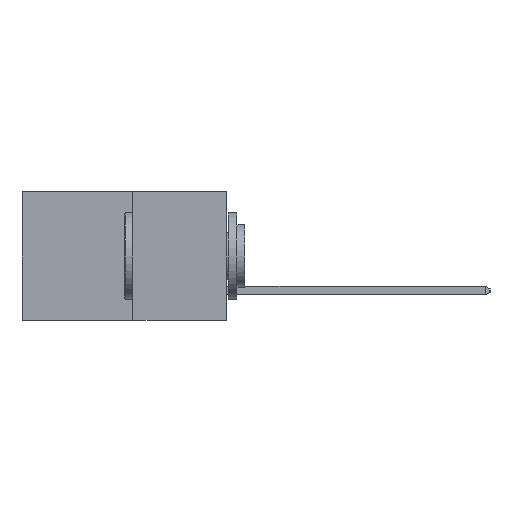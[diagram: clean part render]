
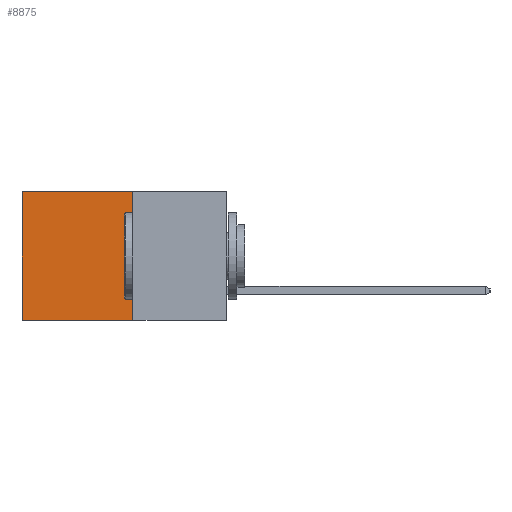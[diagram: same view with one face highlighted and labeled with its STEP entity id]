
A CAD part, left-side view. The second image highlights one B-rep face of the part: STEP entity #8875.
In plain terms, the highlighted planar face has unit normal (-1, 0, 0).
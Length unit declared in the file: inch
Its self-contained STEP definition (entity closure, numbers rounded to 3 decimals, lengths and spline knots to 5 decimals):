
#94 = FACE_OUTER_BOUND ( 'NONE', #8147, .T. ) ;
#225 = VECTOR ( 'NONE', #24396, 39.37008 ) ;
#762 = DIRECTION ( 'NONE',  ( 0., 0., -1. ) ) ;
#2035 = ORIENTED_EDGE ( 'NONE', *, *, #21722, .F. ) ;
#2165 = VERTEX_POINT ( 'NONE', #15482 ) ;
#2166 = LINE ( 'NONE', #13962, #7143 ) ;
#2808 = LINE ( 'NONE', #9241, #24648 ) ;
#4376 = VECTOR ( 'NONE', #4393, 39.37008 ) ;
#4393 = DIRECTION ( 'NONE',  ( 0., 1., 0. ) ) ;
#5026 = LINE ( 'NONE', #23357, #4376 ) ;
#5963 = LINE ( 'NONE', #26495, #225 ) ;
#6356 = DIRECTION ( 'NONE',  ( 0., 0., -1. ) ) ;
#6639 = EDGE_CURVE ( 'NONE', #18866, #8861, #2808, .T. ) ;
#7143 = VECTOR ( 'NONE', #9710, 39.37008 ) ;
#8147 = EDGE_LOOP ( 'NONE', ( #14709, #17660, #2035, #10083 ) ) ;
#8861 = VERTEX_POINT ( 'NONE', #27244 ) ;
#8875 = ADVANCED_FACE ( 'NONE', ( #94 ), #27416, .F. ) ;
#9241 = CARTESIAN_POINT ( 'NONE',  ( 0.277, 0.59, -0.37 ) ) ;
#9710 = DIRECTION ( 'NONE',  ( 0., 0., -1. ) ) ;
#10083 = ORIENTED_EDGE ( 'NONE', *, *, #11048, .T. ) ;
#10363 = CARTESIAN_POINT ( 'NONE',  ( 0.277, 0.27, 0. ) ) ;
#10585 = CARTESIAN_POINT ( 'NONE',  ( 0.277, 0.59, 0. ) ) ;
#11048 = EDGE_CURVE ( 'NONE', #16695, #18866, #5026, .T. ) ;
#12053 = EDGE_CURVE ( 'NONE', #2165, #8861, #5963, .T. ) ;
#12139 = AXIS2_PLACEMENT_3D ( 'NONE', #16864, #19103, #6356 ) ;
#13962 = CARTESIAN_POINT ( 'NONE',  ( 0.277, 0.27, -0.37 ) ) ;
#14709 = ORIENTED_EDGE ( 'NONE', *, *, #6639, .T. ) ;
#15482 = CARTESIAN_POINT ( 'NONE',  ( 0.277, 0.27, -0.37 ) ) ;
#16695 = VERTEX_POINT ( 'NONE', #10363 ) ;
#16864 = CARTESIAN_POINT ( 'NONE',  ( 0.277, 0.27, -0.37 ) ) ;
#17660 = ORIENTED_EDGE ( 'NONE', *, *, #12053, .F. ) ;
#18866 = VERTEX_POINT ( 'NONE', #10585 ) ;
#19103 = DIRECTION ( 'NONE',  ( 1., 0., 0. ) ) ;
#21722 = EDGE_CURVE ( 'NONE', #16695, #2165, #2166, .T. ) ;
#23357 = CARTESIAN_POINT ( 'NONE',  ( 0.277, 0.27, 0. ) ) ;
#24396 = DIRECTION ( 'NONE',  ( 0., 1., 0. ) ) ;
#24648 = VECTOR ( 'NONE', #762, 39.37008 ) ;
#26495 = CARTESIAN_POINT ( 'NONE',  ( 0.277, 0.27, -0.37 ) ) ;
#27244 = CARTESIAN_POINT ( 'NONE',  ( 0.277, 0.59, -0.37 ) ) ;
#27416 = PLANE ( 'NONE',  #12139 ) ;
